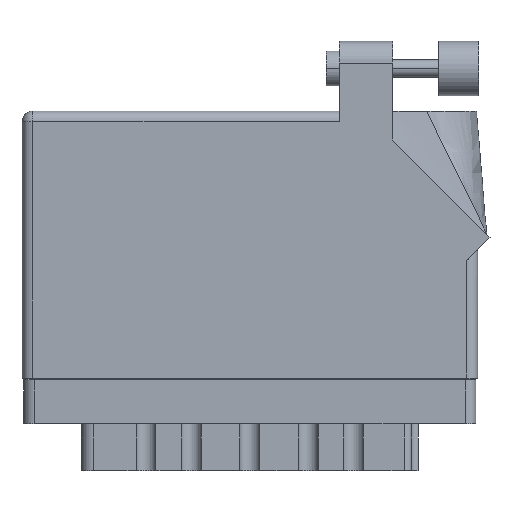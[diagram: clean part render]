
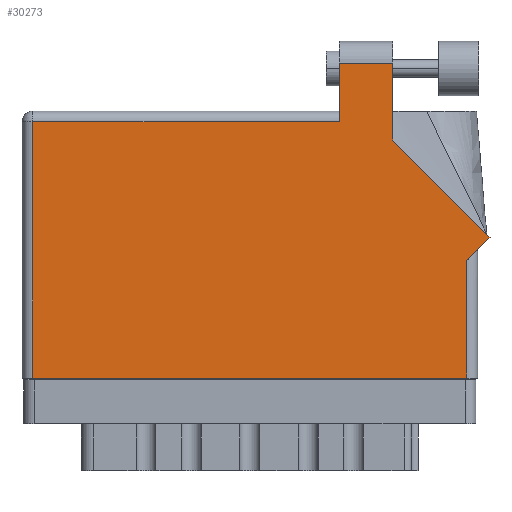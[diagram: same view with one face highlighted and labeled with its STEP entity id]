
A CAD part, front view. The second image highlights one B-rep face of the part: STEP entity #30273.
In plain terms, the highlighted face is planar.
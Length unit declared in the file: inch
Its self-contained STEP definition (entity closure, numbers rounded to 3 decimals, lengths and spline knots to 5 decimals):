
#1062 = CARTESIAN_POINT ( 'NONE',  ( 2.68271, 0.80771, 0. ) ) ;
#2212 = CARTESIAN_POINT ( 'NONE',  ( 0., 0., 0. ) ) ;
#3326 = LINE ( 'NONE', #2212, #45789 ) ;
#3421 = AXIS2_PLACEMENT_3D ( 'NONE', #33149, #6164, #17814 ) ;
#4341 = DIRECTION ( 'NONE',  ( 0., 1., 0. ) ) ;
#4621 = CARTESIAN_POINT ( 'NONE',  ( 2.55, 0.675, 0. ) ) ;
#4758 = ORIENTED_EDGE ( 'NONE', *, *, #45076, .T. ) ;
#4980 = CARTESIAN_POINT ( 'NONE',  ( 2.126, 1.36442, 0. ) ) ;
#5581 = ORIENTED_EDGE ( 'NONE', *, *, #37317, .T. ) ;
#5628 = VECTOR ( 'NONE', #44696, 39.37008 ) ;
#5846 = VERTEX_POINT ( 'NONE', #37188 ) ;
#6164 = DIRECTION ( 'NONE',  ( 0., 0., -1. ) ) ;
#6589 = VECTOR ( 'NONE', #42872, 39.37008 ) ;
#7094 = VECTOR ( 'NONE', #4341, 39.37008 ) ;
#7590 = LINE ( 'NONE', #14870, #42358 ) ;
#7935 = LINE ( 'NONE', #47341, #47475 ) ;
#8379 = EDGE_CURVE ( 'NONE', #43638, #22416, #3326, .T. ) ;
#8916 = ORIENTED_EDGE ( 'NONE', *, *, #16049, .T. ) ;
#9210 = LINE ( 'NONE', #29772, #5628 ) ;
#9271 = CARTESIAN_POINT ( 'NONE',  ( 1.819, 1.468, 0. ) ) ;
#10144 = LINE ( 'NONE', #39036, #6589 ) ;
#10310 = VERTEX_POINT ( 'NONE', #1062 ) ;
#12229 = VERTEX_POINT ( 'NONE', #21966 ) ;
#13335 = CARTESIAN_POINT ( 'NONE',  ( 1.819, 1.53, 0. ) ) ;
#13487 = VERTEX_POINT ( 'NONE', #30539 ) ;
#14222 = CARTESIAN_POINT ( 'NONE',  ( 0.062, 0., 0. ) ) ;
#14870 = CARTESIAN_POINT ( 'NONE',  ( 0., 1.468, 0. ) ) ;
#15172 = EDGE_CURVE ( 'NONE', #12229, #13487, #9210, .T. ) ;
#15253 = DIRECTION ( 'NONE',  ( -0.707, 0.707, 0. ) ) ;
#16049 = EDGE_CURVE ( 'NONE', #22416, #29497, #7935, .T. ) ;
#17430 = EDGE_CURVE ( 'NONE', #29497, #10310, #10144, .T. ) ;
#17814 = DIRECTION ( 'NONE',  ( -1., 0., 0. ) ) ;
#17904 = VECTOR ( 'NONE', #25272, 39.37008 ) ;
#19060 = DIRECTION ( 'NONE',  ( -1., 0., 0. ) ) ;
#20080 = ORIENTED_EDGE ( 'NONE', *, *, #42306, .T. ) ;
#20177 = DIRECTION ( 'NONE',  ( 0., 1., 0. ) ) ;
#21966 = CARTESIAN_POINT ( 'NONE',  ( 2.126, 1.805, 0. ) ) ;
#22416 = VERTEX_POINT ( 'NONE', #40741 ) ;
#23563 = VECTOR ( 'NONE', #31816, 39.37008 ) ;
#25238 = ORIENTED_EDGE ( 'NONE', *, *, #8379, .T. ) ;
#25272 = DIRECTION ( 'NONE',  ( 0., -1., 0. ) ) ;
#26255 = ORIENTED_EDGE ( 'NONE', *, *, #40215, .T. ) ;
#26725 = VERTEX_POINT ( 'NONE', #9271 ) ;
#27461 = LINE ( 'NONE', #4980, #7094 ) ;
#29080 = PLANE ( 'NONE',  #3421 ) ;
#29263 = FACE_OUTER_BOUND ( 'NONE', #29551, .T. ) ;
#29497 = VERTEX_POINT ( 'NONE', #4621 ) ;
#29551 = EDGE_LOOP ( 'NONE', ( #35607, #43517, #5581, #20080, #26255, #25238, #8916, #37322, #4758 ) ) ;
#29772 = CARTESIAN_POINT ( 'NONE',  ( 1.819, 1.805, 0. ) ) ;
#30273 = ADVANCED_FACE ( 'NONE', ( #29263 ), #29080, .F. ) ;
#30341 = VERTEX_POINT ( 'NONE', #41987 ) ;
#30539 = CARTESIAN_POINT ( 'NONE',  ( 1.819, 1.805, 0. ) ) ;
#30606 = EDGE_CURVE ( 'NONE', #30341, #12229, #27461, .T. ) ;
#31816 = DIRECTION ( 'NONE',  ( 0., -1., 0. ) ) ;
#32460 = DIRECTION ( 'NONE',  ( 1., 0., 0. ) ) ;
#33149 = CARTESIAN_POINT ( 'NONE',  ( 0., 1.53, 0. ) ) ;
#33211 = VECTOR ( 'NONE', #15253, 39.37008 ) ;
#35155 = CARTESIAN_POINT ( 'NONE',  ( 2.68271, 0.80771, 0. ) ) ;
#35607 = ORIENTED_EDGE ( 'NONE', *, *, #30606, .T. ) ;
#37188 = CARTESIAN_POINT ( 'NONE',  ( 0.062, 1.468, 0. ) ) ;
#37317 = EDGE_CURVE ( 'NONE', #13487, #26725, #45172, .T. ) ;
#37322 = ORIENTED_EDGE ( 'NONE', *, *, #17430, .T. ) ;
#37425 = LINE ( 'NONE', #35155, #33211 ) ;
#39036 = CARTESIAN_POINT ( 'NONE',  ( 2.612, 0.737, 0. ) ) ;
#40163 = LINE ( 'NONE', #40549, #17904 ) ;
#40215 = EDGE_CURVE ( 'NONE', #5846, #43638, #40163, .T. ) ;
#40549 = CARTESIAN_POINT ( 'NONE',  ( 0.062, 0., 0. ) ) ;
#40741 = CARTESIAN_POINT ( 'NONE',  ( 2.55, 0., 0. ) ) ;
#41987 = CARTESIAN_POINT ( 'NONE',  ( 2.126, 1.36442, 0. ) ) ;
#42306 = EDGE_CURVE ( 'NONE', #26725, #5846, #7590, .T. ) ;
#42358 = VECTOR ( 'NONE', #19060, 39.37008 ) ;
#42872 = DIRECTION ( 'NONE',  ( 0.707, 0.707, 0. ) ) ;
#43517 = ORIENTED_EDGE ( 'NONE', *, *, #15172, .T. ) ;
#43638 = VERTEX_POINT ( 'NONE', #14222 ) ;
#44696 = DIRECTION ( 'NONE',  ( -1., 0., 0. ) ) ;
#45076 = EDGE_CURVE ( 'NONE', #10310, #30341, #37425, .T. ) ;
#45172 = LINE ( 'NONE', #13335, #23563 ) ;
#45789 = VECTOR ( 'NONE', #32460, 39.37008 ) ;
#47341 = CARTESIAN_POINT ( 'NONE',  ( 2.55, 0.737, 0. ) ) ;
#47475 = VECTOR ( 'NONE', #20177, 39.37008 ) ;
